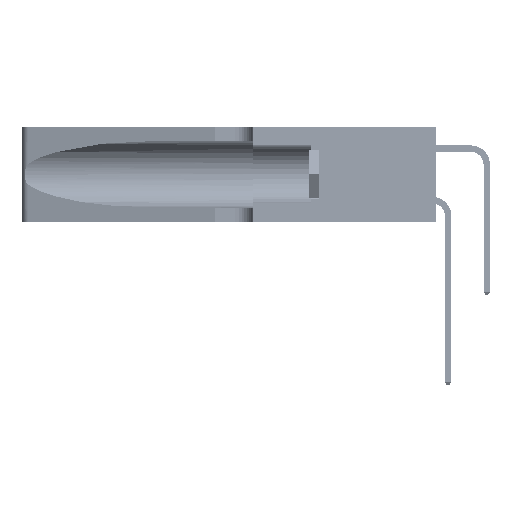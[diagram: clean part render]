
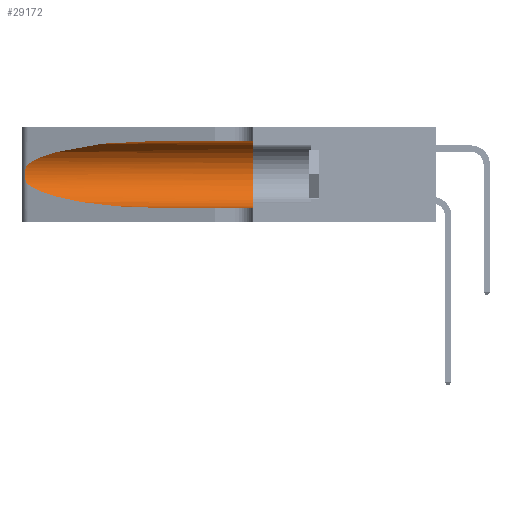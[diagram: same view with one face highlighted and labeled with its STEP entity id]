
A CAD part, left-side view. The second image highlights one B-rep face of the part: STEP entity #29172.
In plain terms, the highlighted cylindrical face has radius 3.308 mm (diameter 6.617 mm), a partial arc.
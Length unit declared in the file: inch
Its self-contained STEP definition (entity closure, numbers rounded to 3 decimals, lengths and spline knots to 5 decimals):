
#62 = CARTESIAN_POINT ( 'NONE',  ( 0.26018, 1.23835, 0.19895 ) ) ;
#136 = VERTEX_POINT ( 'NONE', #47076 ) ;
#2027 = CARTESIAN_POINT ( 'NONE',  ( 0.1305, 0.72297, 0.05475 ) ) ;
#4470 = CARTESIAN_POINT ( 'NONE',  ( 0.26075, 1.23896, 0.178 ) ) ;
#4931 = CARTESIAN_POINT ( 'NONE',  ( 0.18966, 0.96281, 0.31525 ) ) ;
#5015 = CARTESIAN_POINT ( 'NONE',  ( 0.2373, 1.15595, 0.08982 ) ) ;
#6542 = EDGE_CURVE ( 'NONE', #17977, #136, #7686, .T. ) ;
#6698 = VECTOR ( 'NONE', #9358, 39.37008 ) ;
#7686 = LINE ( 'NONE', #43378, #29236 ) ;
#8585 = AXIS2_PLACEMENT_3D ( 'NONE', #47717, #22063, #52040 ) ;
#8839 = CARTESIAN_POINT ( 'NONE',  ( 0.25856, 1.23593, 0.16098 ) ) ;
#9202 = EDGE_CURVE ( 'NONE', #17977, #39291, #41412, .T. ) ;
#9358 = DIRECTION ( 'NONE',  ( 0., -1., 0. ) ) ;
#9377 = CARTESIAN_POINT ( 'NONE',  ( 0.18966, 0.96281, 0.05475 ) ) ;
#9636 = CARTESIAN_POINT ( 'NONE',  ( 0.1305, 1.61858, 0.185 ) ) ;
#13159 = CARTESIAN_POINT ( 'NONE',  ( 0.25639, 1.23186, 0.15144 ) ) ;
#13333 = EDGE_LOOP ( 'NONE', ( #24881, #30286, #38719, #55540, #34122, #35901 ) ) ;
#13619 = CARTESIAN_POINT ( 'NONE',  ( 0.25487, 1.22718, 0.22369 ) ) ;
#13785 = DIRECTION ( 'NONE',  ( 0., 0., -1. ) ) ;
#13971 = DIRECTION ( 'NONE',  ( 0., -1., 0. ) ) ;
#17400 = EDGE_CURVE ( 'NONE', #18931, #32777, #51075, .T. ) ;
#17514 = CARTESIAN_POINT ( 'NONE',  ( 0.25487, 1.22718, 0.14631 ) ) ;
#17660 = DIRECTION ( 'NONE',  ( 0., -1., 0. ) ) ;
#17977 = VERTEX_POINT ( 'NONE', #52135 ) ;
#18931 = VERTEX_POINT ( 'NONE', #2027 ) ;
#21681 = CARTESIAN_POINT ( 'NONE',  ( 0.25639, 1.23184, 0.21858 ) ) ;
#22063 = DIRECTION ( 'NONE',  ( 0., 1., 0. ) ) ;
#24881 = ORIENTED_EDGE ( 'NONE', *, *, #9202, .T. ) ;
#26004 = CARTESIAN_POINT ( 'NONE',  ( 0.25854, 1.2359, 0.20912 ) ) ;
#26322 = CARTESIAN_POINT ( 'NONE',  ( 0.25487, 1.22718, 0.22369 ) ) ;
#26389 = CARTESIAN_POINT ( 'NONE',  ( 0.1305, 0.35, 0.05475 ) ) ;
#26814 = EDGE_CURVE ( 'NONE', #46338, #18931, #53104, .T. ) ;
#27086 = CARTESIAN_POINT ( 'NONE',  ( 0.25487, 1.22718, 0.14631 ) ) ;
#27804 = CIRCLE ( 'NONE', #8585, 0.13025 ) ;
#29172 = ADVANCED_FACE ( 'NONE', ( #41436 ), #30023, .F. ) ;
#29236 = VECTOR ( 'NONE', #17660, 39.37008 ) ;
#30023 = CYLINDRICAL_SURFACE ( 'NONE', #33869, 0.13025 ) ;
#30280 = CARTESIAN_POINT ( 'NONE',  ( 0.26075, 1.23896, 0.19203 ) ) ;
#30286 = ORIENTED_EDGE ( 'NONE', *, *, #34667, .T. ) ;
#30729 = CARTESIAN_POINT ( 'NONE',  ( 0.2373, 1.15595, 0.28018 ) ) ;
#32777 = VERTEX_POINT ( 'NONE', #26389 ) ;
#33151 = B_SPLINE_CURVE_WITH_KNOTS ( 'NONE', 3,
 ( #43040, #47343, #21681, #51658, #26004, #62, #30280, #4470, #34599, #8839, #38924, #13159, #43230, #17514 ),
 .UNSPECIFIED., .F., .F.,
 ( 4, 2, 2, 2, 2, 2, 4 ),
 ( 0., 0.00027, 0.00053, 0.00107, 0.0016, 0.00187, 0.00214 ),
 .UNSPECIFIED. ) ;
#33869 = AXIS2_PLACEMENT_3D ( 'NONE', #9636, #13971, #13785 ) ;
#34122 = ORIENTED_EDGE ( 'NONE', *, *, #38537, .F. ) ;
#34599 = CARTESIAN_POINT ( 'NONE',  ( 0.26017, 1.23833, 0.17102 ) ) ;
#34667 = EDGE_CURVE ( 'NONE', #39291, #46338, #33151, .T. ) ;
#35128 = CARTESIAN_POINT ( 'NONE',  ( 0.1305, 1.61858, 0.05475 ) ) ;
#35901 = ORIENTED_EDGE ( 'NONE', *, *, #6542, .F. ) ;
#38537 = EDGE_CURVE ( 'NONE', #136, #32777, #27804, .T. ) ;
#38719 = ORIENTED_EDGE ( 'NONE', *, *, #26814, .T. ) ;
#38924 = CARTESIAN_POINT ( 'NONE',  ( 0.25789, 1.23486, 0.15765 ) ) ;
#39291 = VERTEX_POINT ( 'NONE', #26322 ) ;
#39378 = CARTESIAN_POINT ( 'NONE',  ( 0.1305, 0.72297, 0.31525 ) ) ;
#39465 = CARTESIAN_POINT ( 'NONE',  ( 0.1305, 0.72297, 0.05475 ) ) ;
#41412 =( BOUNDED_CURVE ( )  B_SPLINE_CURVE ( 3, ( #39378, #4931, #30729, #13619 ),
 .UNSPECIFIED., .F., .F. ) 
 B_SPLINE_CURVE_WITH_KNOTS ( ( 4, 4 ),
 ( 1.5708, 2.84003 ),
 .UNSPECIFIED. ) 
 CURVE ( )  GEOMETRIC_REPRESENTATION_ITEM ( )  RATIONAL_B_SPLINE_CURVE ( ( 1., 0.87, 0.87, 1. ) ) 
 REPRESENTATION_ITEM ( '' )  );
#41436 = FACE_OUTER_BOUND ( 'NONE', #13333, .T. ) ;
#43040 = CARTESIAN_POINT ( 'NONE',  ( 0.25487, 1.22718, 0.22369 ) ) ;
#43230 = CARTESIAN_POINT ( 'NONE',  ( 0.25555, 1.22993, 0.14849 ) ) ;
#43378 = CARTESIAN_POINT ( 'NONE',  ( 0.1305, 1.61858, 0.31525 ) ) ;
#46338 = VERTEX_POINT ( 'NONE', #27086 ) ;
#47076 = CARTESIAN_POINT ( 'NONE',  ( 0.1305, 0.35, 0.31525 ) ) ;
#47343 = CARTESIAN_POINT ( 'NONE',  ( 0.25555, 1.22994, 0.2215 ) ) ;
#47717 = CARTESIAN_POINT ( 'NONE',  ( 0.1305, 0.35, 0.185 ) ) ;
#47883 = CARTESIAN_POINT ( 'NONE',  ( 0.25487, 1.22718, 0.14631 ) ) ;
#51075 = LINE ( 'NONE', #35128, #6698 ) ;
#51658 = CARTESIAN_POINT ( 'NONE',  ( 0.25787, 1.23484, 0.2124 ) ) ;
#52040 = DIRECTION ( 'NONE',  ( 0., 0., 1. ) ) ;
#52135 = CARTESIAN_POINT ( 'NONE',  ( 0.1305, 0.72297, 0.31525 ) ) ;
#53104 =( BOUNDED_CURVE ( )  B_SPLINE_CURVE ( 3, ( #47883, #5015, #9377, #39465 ),
 .UNSPECIFIED., .F., .F. ) 
 B_SPLINE_CURVE_WITH_KNOTS ( ( 4, 4 ),
 ( 3.44316, 4.71239 ),
 .UNSPECIFIED. ) 
 CURVE ( )  GEOMETRIC_REPRESENTATION_ITEM ( )  RATIONAL_B_SPLINE_CURVE ( ( 1., 0.87, 0.87, 1. ) ) 
 REPRESENTATION_ITEM ( '' )  );
#55540 = ORIENTED_EDGE ( 'NONE', *, *, #17400, .T. ) ;
